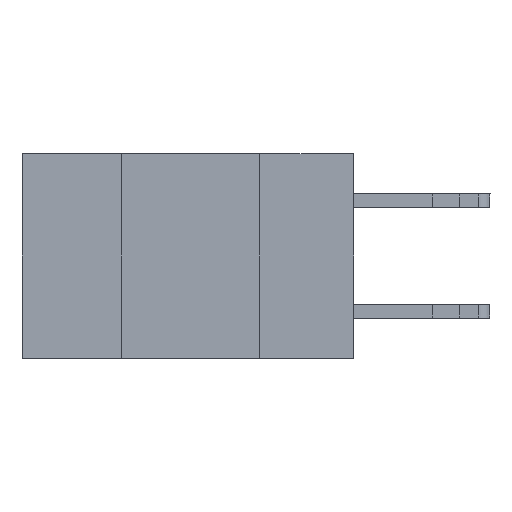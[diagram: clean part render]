
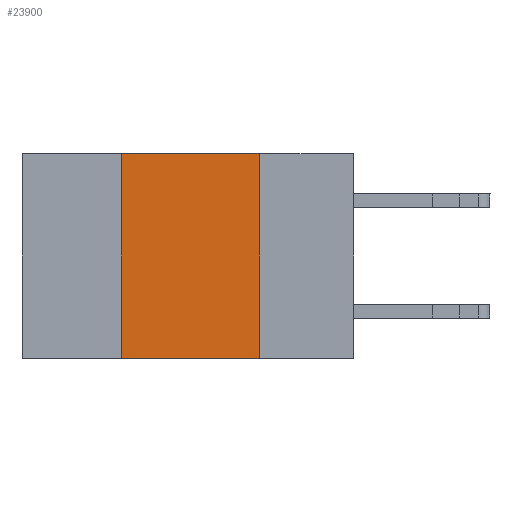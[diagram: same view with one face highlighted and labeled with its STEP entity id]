
A CAD part, left-side view. The second image highlights one B-rep face of the part: STEP entity #23900.
In plain terms, the highlighted planar face has unit normal (-1, 0, 0).
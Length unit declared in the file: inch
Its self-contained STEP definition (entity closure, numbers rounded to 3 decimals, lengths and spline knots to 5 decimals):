
#906 = CARTESIAN_POINT ( 'NONE',  ( 0., 0.6, -0.37 ) ) ;
#1086 = CARTESIAN_POINT ( 'NONE',  ( 0., 0.42, 0. ) ) ;
#1112 = VECTOR ( 'NONE', #4993, 39.37008 ) ;
#1118 = CARTESIAN_POINT ( 'NONE',  ( 0., 0.6, 0. ) ) ;
#2082 = VECTOR ( 'NONE', #14578, 39.37008 ) ;
#2980 = EDGE_CURVE ( 'NONE', #20489, #27455, #14202, .T. ) ;
#3271 = LINE ( 'NONE', #1086, #5220 ) ;
#4099 = FACE_OUTER_BOUND ( 'NONE', #26721, .T. ) ;
#4732 = VERTEX_POINT ( 'NONE', #22072 ) ;
#4993 = DIRECTION ( 'NONE',  ( 0., 0., -1. ) ) ;
#5220 = VECTOR ( 'NONE', #18905, 39.37008 ) ;
#5577 = DIRECTION ( 'NONE',  ( 0., -1., 0. ) ) ;
#7519 = CARTESIAN_POINT ( 'NONE',  ( 0., 0.17, -0.37 ) ) ;
#7750 = VERTEX_POINT ( 'NONE', #22282 ) ;
#8278 = LINE ( 'NONE', #1118, #2082 ) ;
#9740 = ORIENTED_EDGE ( 'NONE', *, *, #2980, .F. ) ;
#10115 = ORIENTED_EDGE ( 'NONE', *, *, #27002, .T. ) ;
#11878 = LINE ( 'NONE', #906, #15103 ) ;
#14202 = LINE ( 'NONE', #20493, #1112 ) ;
#14578 = DIRECTION ( 'NONE',  ( 0., -1., 0. ) ) ;
#15103 = VECTOR ( 'NONE', #5577, 39.37008 ) ;
#17813 = DIRECTION ( 'NONE',  ( 1., 0., 0. ) ) ;
#18905 = DIRECTION ( 'NONE',  ( 0., 0., 1. ) ) ;
#19578 = DIRECTION ( 'NONE',  ( 0., 0., -1. ) ) ;
#20300 = ORIENTED_EDGE ( 'NONE', *, *, #25217, .F. ) ;
#20489 = VERTEX_POINT ( 'NONE', #24506 ) ;
#20493 = CARTESIAN_POINT ( 'NONE',  ( 0., 0.17, 0. ) ) ;
#21652 = CARTESIAN_POINT ( 'NONE',  ( 0., 0.6, 0. ) ) ;
#22072 = CARTESIAN_POINT ( 'NONE',  ( 0., 0.42, 0. ) ) ;
#22282 = CARTESIAN_POINT ( 'NONE',  ( 0., 0.42, -0.37 ) ) ;
#22917 = AXIS2_PLACEMENT_3D ( 'NONE', #21652, #17813, #19578 ) ;
#23900 = ADVANCED_FACE ( 'NONE', ( #4099 ), #28831, .F. ) ;
#24506 = CARTESIAN_POINT ( 'NONE',  ( 0., 0.17, 0. ) ) ;
#25217 = EDGE_CURVE ( 'NONE', #7750, #4732, #3271, .T. ) ;
#26721 = EDGE_LOOP ( 'NONE', ( #9740, #28166, #20300, #10115 ) ) ;
#27002 = EDGE_CURVE ( 'NONE', #7750, #27455, #11878, .T. ) ;
#27455 = VERTEX_POINT ( 'NONE', #7519 ) ;
#28166 = ORIENTED_EDGE ( 'NONE', *, *, #28269, .F. ) ;
#28269 = EDGE_CURVE ( 'NONE', #4732, #20489, #8278, .T. ) ;
#28831 = PLANE ( 'NONE',  #22917 ) ;
